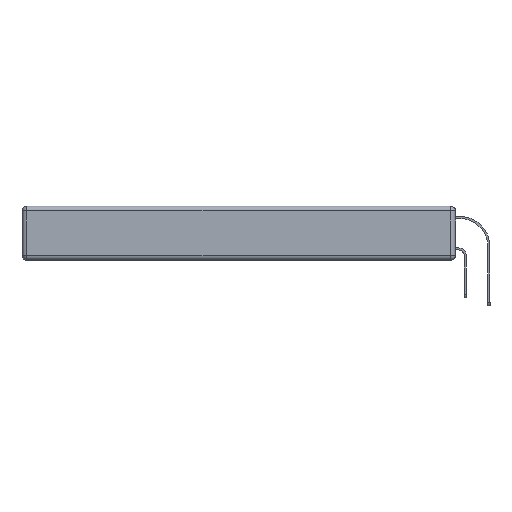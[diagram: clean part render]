
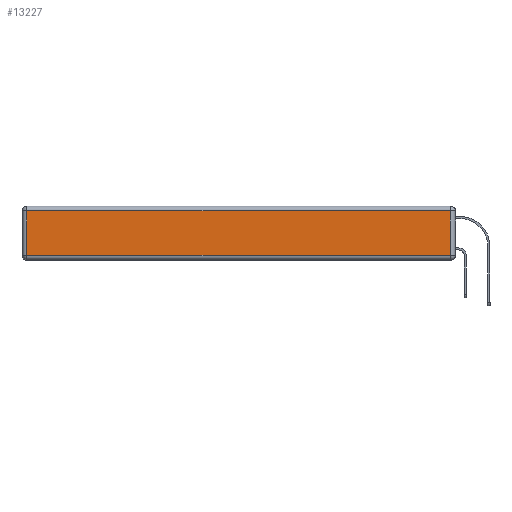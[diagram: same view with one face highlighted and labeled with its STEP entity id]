
A CAD part, left-side view. The second image highlights one B-rep face of the part: STEP entity #13227.
In plain terms, the highlighted planar face has unit normal (-1, 0, 0).
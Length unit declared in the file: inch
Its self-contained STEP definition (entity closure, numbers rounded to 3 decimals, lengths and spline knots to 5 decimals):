
#198 = AXIS2_PLACEMENT_3D ( 'NONE', #12977, #11631, #9315 ) ;
#313 = CARTESIAN_POINT ( 'NONE',  ( 0., 0., -0.313 ) ) ;
#518 = DIRECTION ( 'NONE',  ( 0., 0., 1. ) ) ;
#648 = ORIENTED_EDGE ( 'NONE', *, *, #10862, .T. ) ;
#2491 = DIRECTION ( 'NONE',  ( 0., 0., -1. ) ) ;
#3386 = CARTESIAN_POINT ( 'NONE',  ( 0., 2.72, -0.343 ) ) ;
#3596 = VECTOR ( 'NONE', #518, 39.37008 ) ;
#3839 = EDGE_CURVE ( 'NONE', #3983, #14536, #11666, .T. ) ;
#3940 = LINE ( 'NONE', #12924, #3596 ) ;
#3983 = VERTEX_POINT ( 'NONE', #6207 ) ;
#4218 = CARTESIAN_POINT ( 'NONE',  ( 0., 0.03, -0.03 ) ) ;
#4346 = CARTESIAN_POINT ( 'NONE',  ( 0., 0.03, -0.313 ) ) ;
#4577 = LINE ( 'NONE', #3386, #7385 ) ;
#4750 = FACE_OUTER_BOUND ( 'NONE', #10960, .T. ) ;
#4864 = DIRECTION ( 'NONE',  ( 0., -1., 0. ) ) ;
#5519 = ORIENTED_EDGE ( 'NONE', *, *, #14146, .T. ) ;
#5675 = CARTESIAN_POINT ( 'NONE',  ( 0., 2.75, -0.03 ) ) ;
#5689 = ORIENTED_EDGE ( 'NONE', *, *, #3839, .T. ) ;
#6207 = CARTESIAN_POINT ( 'NONE',  ( 0., 2.72, -0.313 ) ) ;
#7385 = VECTOR ( 'NONE', #2491, 39.37008 ) ;
#7570 = VECTOR ( 'NONE', #4864, 39.37008 ) ;
#8444 = VERTEX_POINT ( 'NONE', #14196 ) ;
#9000 = EDGE_CURVE ( 'NONE', #14536, #9859, #3940, .T. ) ;
#9040 = DIRECTION ( 'NONE',  ( 0., 1., 0. ) ) ;
#9315 = DIRECTION ( 'NONE',  ( 0., 0., 1. ) ) ;
#9859 = VERTEX_POINT ( 'NONE', #4218 ) ;
#10862 = EDGE_CURVE ( 'NONE', #9859, #8444, #11519, .T. ) ;
#10903 = ORIENTED_EDGE ( 'NONE', *, *, #9000, .T. ) ;
#10960 = EDGE_LOOP ( 'NONE', ( #5689, #10903, #648, #5519 ) ) ;
#11519 = LINE ( 'NONE', #5675, #14705 ) ;
#11631 = DIRECTION ( 'NONE',  ( -1., 0., 0. ) ) ;
#11666 = LINE ( 'NONE', #313, #7570 ) ;
#12924 = CARTESIAN_POINT ( 'NONE',  ( 0., 0.03, -0.343 ) ) ;
#12977 = CARTESIAN_POINT ( 'NONE',  ( 0., 0., -0.343 ) ) ;
#13227 = ADVANCED_FACE ( 'NONE', ( #4750 ), #14096, .T. ) ;
#14096 = PLANE ( 'NONE',  #198 ) ;
#14146 = EDGE_CURVE ( 'NONE', #8444, #3983, #4577, .T. ) ;
#14196 = CARTESIAN_POINT ( 'NONE',  ( 0., 2.72, -0.03 ) ) ;
#14536 = VERTEX_POINT ( 'NONE', #4346 ) ;
#14705 = VECTOR ( 'NONE', #9040, 39.37008 ) ;
